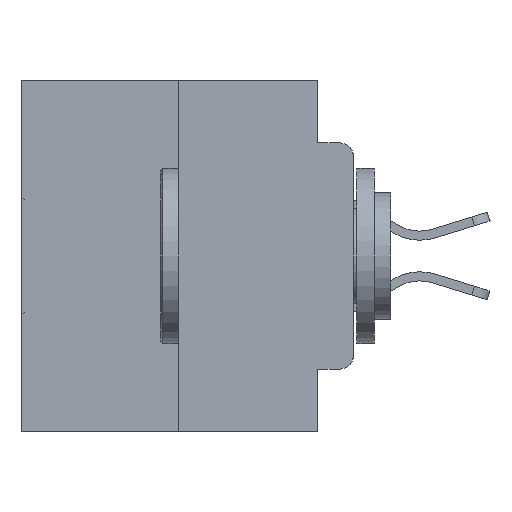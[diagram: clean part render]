
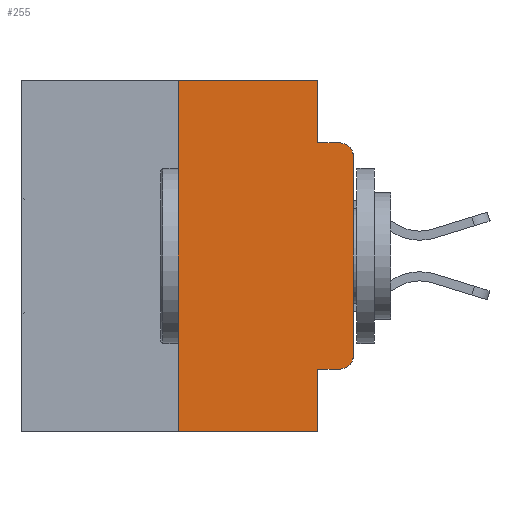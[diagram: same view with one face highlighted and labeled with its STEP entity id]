
A CAD part, left-side view. The second image highlights one B-rep face of the part: STEP entity #255.
In plain terms, the highlighted planar face has unit normal (-1, 0, 0).
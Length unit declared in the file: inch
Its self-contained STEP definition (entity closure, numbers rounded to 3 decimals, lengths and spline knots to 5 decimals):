
#25 = ORIENTED_EDGE ( 'NONE', *, *, #22458, .T. ) ;
#255 = ADVANCED_FACE ( 'NONE', ( #24141 ), #29078, .F. ) ;
#511 = CARTESIAN_POINT ( 'NONE',  ( 0., 0.051, 0. ) ) ;
#1575 = DIRECTION ( 'NONE',  ( 0., -1., 0. ) ) ;
#2596 = VERTEX_POINT ( 'NONE', #17938 ) ;
#2735 = DIRECTION ( 'NONE',  ( 0., -1., 0. ) ) ;
#2872 = CIRCLE ( 'NONE', #22771, 0.02 ) ;
#3143 = LINE ( 'NONE', #8811, #28081 ) ;
#3295 = ORIENTED_EDGE ( 'NONE', *, *, #12356, .F. ) ;
#4154 = EDGE_CURVE ( 'NONE', #2596, #30941, #28071, .T. ) ;
#4568 = EDGE_LOOP ( 'NONE', ( #26767, #9109, #3295, #16311, #23566, #18734, #25, #6556, #20222, #26559 ) ) ;
#4911 = VERTEX_POINT ( 'NONE', #27476 ) ;
#5248 = CARTESIAN_POINT ( 'NONE',  ( 0., 0.473, -0.5 ) ) ;
#5285 = VECTOR ( 'NONE', #15527, 39.37008 ) ;
#5813 = EDGE_CURVE ( 'NONE', #25147, #2596, #7343, .T. ) ;
#6275 = VERTEX_POINT ( 'NONE', #23248 ) ;
#6556 = ORIENTED_EDGE ( 'NONE', *, *, #7491, .F. ) ;
#6561 = VECTOR ( 'NONE', #30902, 39.37008 ) ;
#7343 = LINE ( 'NONE', #14435, #6561 ) ;
#7452 = DIRECTION ( 'NONE',  ( -1., 0., 0. ) ) ;
#7491 = EDGE_CURVE ( 'NONE', #25147, #13763, #30846, .T. ) ;
#7638 = VECTOR ( 'NONE', #27960, 39.37008 ) ;
#7956 = VERTEX_POINT ( 'NONE', #18984 ) ;
#8139 = AXIS2_PLACEMENT_3D ( 'NONE', #10999, #29322, #29173 ) ;
#8811 = CARTESIAN_POINT ( 'NONE',  ( 0., 0., 0. ) ) ;
#9109 = ORIENTED_EDGE ( 'NONE', *, *, #15629, .T. ) ;
#9140 = EDGE_CURVE ( 'NONE', #17433, #6275, #26841, .T. ) ;
#9323 = VECTOR ( 'NONE', #2735, 39.37008 ) ;
#9858 = CARTESIAN_POINT ( 'NONE',  ( 0., 0.25, -0.5 ) ) ;
#10361 = DIRECTION ( 'NONE',  ( 0., 0., -1. ) ) ;
#10745 = EDGE_CURVE ( 'NONE', #22303, #4911, #19280, .T. ) ;
#10999 = CARTESIAN_POINT ( 'NONE',  ( 0., 0.473, 0. ) ) ;
#11720 = VECTOR ( 'NONE', #27002, 39.37008 ) ;
#12168 = CARTESIAN_POINT ( 'NONE',  ( 0., 0.02, -0.1085 ) ) ;
#12356 = EDGE_CURVE ( 'NONE', #4911, #13006, #29921, .T. ) ;
#12377 = CARTESIAN_POINT ( 'NONE',  ( 0., 0.473, 0. ) ) ;
#12499 = CARTESIAN_POINT ( 'NONE',  ( 0., 0.051, -0.5 ) ) ;
#12655 = CARTESIAN_POINT ( 'NONE',  ( 0., 0., -0.3915 ) ) ;
#13006 = VERTEX_POINT ( 'NONE', #23477 ) ;
#13743 = CARTESIAN_POINT ( 'NONE',  ( 0., 0.051, -0.0885 ) ) ;
#13763 = VERTEX_POINT ( 'NONE', #12499 ) ;
#14321 = CARTESIAN_POINT ( 'NONE',  ( 0., 0.051, 0. ) ) ;
#14435 = CARTESIAN_POINT ( 'NONE',  ( 0., 0.051, -0.4115 ) ) ;
#14600 = DIRECTION ( 'NONE',  ( 0., 0., -1. ) ) ;
#15527 = DIRECTION ( 'NONE',  ( 0., 0., -1. ) ) ;
#15629 = EDGE_CURVE ( 'NONE', #7956, #13006, #2872, .T. ) ;
#16311 = ORIENTED_EDGE ( 'NONE', *, *, #10745, .F. ) ;
#17256 = EDGE_CURVE ( 'NONE', #30941, #7956, #3143, .T. ) ;
#17433 = VERTEX_POINT ( 'NONE', #9858 ) ;
#17484 = EDGE_CURVE ( 'NONE', #6275, #22303, #29178, .T. ) ;
#17938 = CARTESIAN_POINT ( 'NONE',  ( 0., 0.02, -0.4115 ) ) ;
#18179 = LINE ( 'NONE', #5248, #11720 ) ;
#18541 = VECTOR ( 'NONE', #10361, 39.37008 ) ;
#18547 = DIRECTION ( 'NONE',  ( 0., 0., 1. ) ) ;
#18734 = ORIENTED_EDGE ( 'NONE', *, *, #9140, .F. ) ;
#18984 = CARTESIAN_POINT ( 'NONE',  ( 0., 0., -0.1085 ) ) ;
#19280 = LINE ( 'NONE', #511, #18541 ) ;
#20222 = ORIENTED_EDGE ( 'NONE', *, *, #5813, .T. ) ;
#21576 = CARTESIAN_POINT ( 'NONE',  ( 0., 0.051, -0.4115 ) ) ;
#21909 = CARTESIAN_POINT ( 'NONE',  ( 0., 0.02, -0.3915 ) ) ;
#22303 = VERTEX_POINT ( 'NONE', #14321 ) ;
#22458 = EDGE_CURVE ( 'NONE', #17433, #13763, #18179, .T. ) ;
#22771 = AXIS2_PLACEMENT_3D ( 'NONE', #12168, #28916, #14600 ) ;
#23248 = CARTESIAN_POINT ( 'NONE',  ( 0., 0.25, 0. ) ) ;
#23477 = CARTESIAN_POINT ( 'NONE',  ( 0., 0.02, -0.0885 ) ) ;
#23566 = ORIENTED_EDGE ( 'NONE', *, *, #17484, .F. ) ;
#23649 = VECTOR ( 'NONE', #1575, 39.37008 ) ;
#24141 = FACE_OUTER_BOUND ( 'NONE', #4568, .T. ) ;
#24311 = DIRECTION ( 'NONE',  ( 0., 0., -1. ) ) ;
#25147 = VERTEX_POINT ( 'NONE', #21576 ) ;
#26559 = ORIENTED_EDGE ( 'NONE', *, *, #4154, .T. ) ;
#26767 = ORIENTED_EDGE ( 'NONE', *, *, #17256, .T. ) ;
#26841 = LINE ( 'NONE', #30313, #7638 ) ;
#27002 = DIRECTION ( 'NONE',  ( 0., -1., 0. ) ) ;
#27445 = CARTESIAN_POINT ( 'NONE',  ( 0., 0.051, 0. ) ) ;
#27476 = CARTESIAN_POINT ( 'NONE',  ( 0., 0.051, -0.0885 ) ) ;
#27960 = DIRECTION ( 'NONE',  ( 0., 0., 1. ) ) ;
#28071 = CIRCLE ( 'NONE', #28299, 0.02 ) ;
#28081 = VECTOR ( 'NONE', #18547, 39.37008 ) ;
#28299 = AXIS2_PLACEMENT_3D ( 'NONE', #21909, #7452, #24311 ) ;
#28916 = DIRECTION ( 'NONE',  ( -1., 0., 0. ) ) ;
#29078 = PLANE ( 'NONE',  #8139 ) ;
#29173 = DIRECTION ( 'NONE',  ( 0., 0., -1. ) ) ;
#29178 = LINE ( 'NONE', #12377, #9323 ) ;
#29322 = DIRECTION ( 'NONE',  ( 1., 0., 0. ) ) ;
#29921 = LINE ( 'NONE', #13743, #23649 ) ;
#30313 = CARTESIAN_POINT ( 'NONE',  ( 0., 0.25, 0. ) ) ;
#30846 = LINE ( 'NONE', #27445, #5285 ) ;
#30902 = DIRECTION ( 'NONE',  ( 0., -1., 0. ) ) ;
#30941 = VERTEX_POINT ( 'NONE', #12655 ) ;
